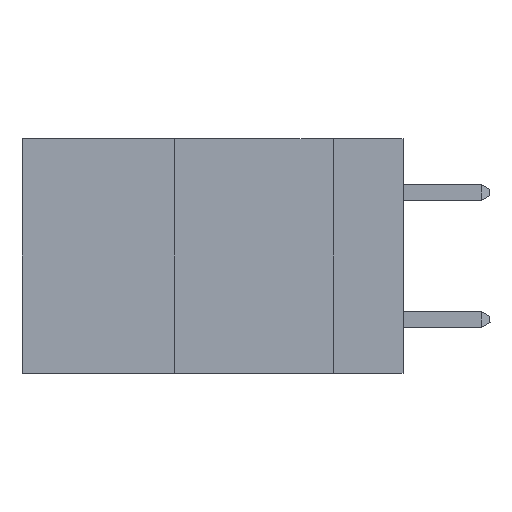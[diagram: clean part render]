
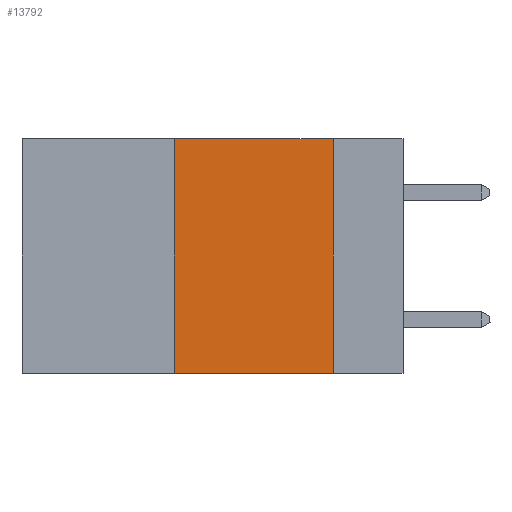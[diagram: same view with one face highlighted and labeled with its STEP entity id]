
A CAD part, left-side view. The second image highlights one B-rep face of the part: STEP entity #13792.
In plain terms, the highlighted planar face has unit normal (-1, 0, 0).
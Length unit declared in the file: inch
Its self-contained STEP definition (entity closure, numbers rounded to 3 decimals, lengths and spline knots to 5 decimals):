
#3272 = ORIENTED_EDGE ( 'NONE', *, *, #7918, .F. ) ;
#3753 = CARTESIAN_POINT ( 'NONE',  ( 0., 0.6, 0. ) ) ;
#4464 = LINE ( 'NONE', #36418, #12197 ) ;
#4474 = CARTESIAN_POINT ( 'NONE',  ( 0., 0.11, 0. ) ) ;
#4761 = VERTEX_POINT ( 'NONE', #7314 ) ;
#6375 = DIRECTION ( 'NONE',  ( 0., 0., -1. ) ) ;
#7314 = CARTESIAN_POINT ( 'NONE',  ( 0., 0.36, -0.37 ) ) ;
#7918 = EDGE_CURVE ( 'NONE', #14280, #40256, #25761, .T. ) ;
#8118 = DIRECTION ( 'NONE',  ( 0., 0., 1. ) ) ;
#9967 = DIRECTION ( 'NONE',  ( 0., -1., 0. ) ) ;
#12197 = VECTOR ( 'NONE', #9967, 39.37008 ) ;
#13792 = ADVANCED_FACE ( 'NONE', ( #39382 ), #28399, .F. ) ;
#14280 = VERTEX_POINT ( 'NONE', #4474 ) ;
#14662 = LINE ( 'NONE', #3753, #30195 ) ;
#15890 = VECTOR ( 'NONE', #6375, 39.37008 ) ;
#16644 = EDGE_LOOP ( 'NONE', ( #3272, #29649, #23956, #25007 ) ) ;
#18505 = DIRECTION ( 'NONE',  ( 1., 0., 0. ) ) ;
#19891 = CARTESIAN_POINT ( 'NONE',  ( 0., 0.36, 0. ) ) ;
#23627 = VECTOR ( 'NONE', #8118, 39.37008 ) ;
#23956 = ORIENTED_EDGE ( 'NONE', *, *, #28809, .F. ) ;
#25007 = ORIENTED_EDGE ( 'NONE', *, *, #29062, .T. ) ;
#25761 = LINE ( 'NONE', #39297, #15890 ) ;
#28399 = PLANE ( 'NONE',  #31025 ) ;
#28809 = EDGE_CURVE ( 'NONE', #4761, #39556, #31391, .T. ) ;
#29062 = EDGE_CURVE ( 'NONE', #4761, #40256, #4464, .T. ) ;
#29649 = ORIENTED_EDGE ( 'NONE', *, *, #39599, .F. ) ;
#30195 = VECTOR ( 'NONE', #36683, 39.37008 ) ;
#30604 = CARTESIAN_POINT ( 'NONE',  ( 0., 0.11, -0.37 ) ) ;
#31025 = AXIS2_PLACEMENT_3D ( 'NONE', #34997, #18505, #41592 ) ;
#31391 = LINE ( 'NONE', #40996, #23627 ) ;
#34997 = CARTESIAN_POINT ( 'NONE',  ( 0., 0.6, 0. ) ) ;
#36418 = CARTESIAN_POINT ( 'NONE',  ( 0., 0.6, -0.37 ) ) ;
#36683 = DIRECTION ( 'NONE',  ( 0., -1., 0. ) ) ;
#39297 = CARTESIAN_POINT ( 'NONE',  ( 0., 0.11, 0. ) ) ;
#39382 = FACE_OUTER_BOUND ( 'NONE', #16644, .T. ) ;
#39556 = VERTEX_POINT ( 'NONE', #19891 ) ;
#39599 = EDGE_CURVE ( 'NONE', #39556, #14280, #14662, .T. ) ;
#40256 = VERTEX_POINT ( 'NONE', #30604 ) ;
#40996 = CARTESIAN_POINT ( 'NONE',  ( 0., 0.36, 0. ) ) ;
#41592 = DIRECTION ( 'NONE',  ( 0., 0., -1. ) ) ;
